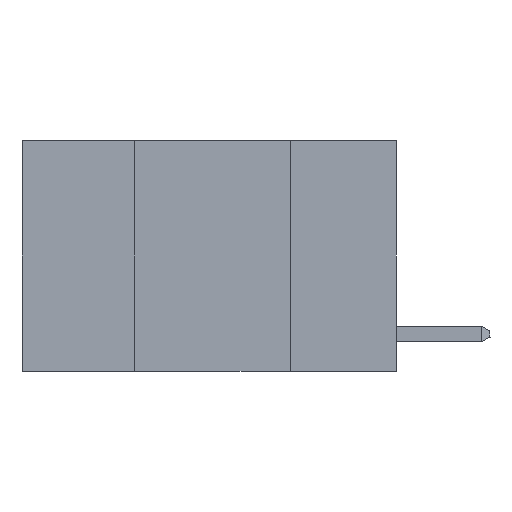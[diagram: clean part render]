
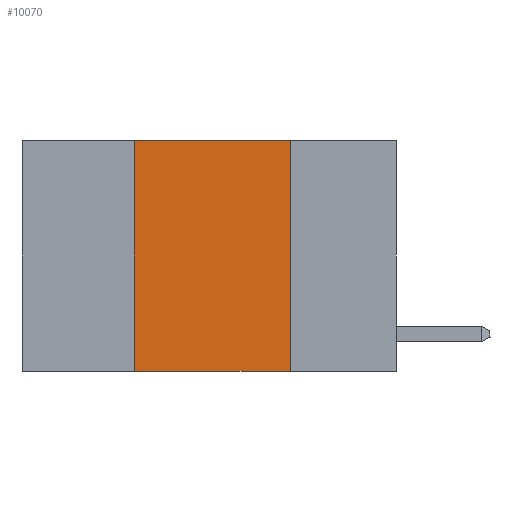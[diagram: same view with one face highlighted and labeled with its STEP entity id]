
A CAD part, left-side view. The second image highlights one B-rep face of the part: STEP entity #10070.
In plain terms, the highlighted planar face has unit normal (-1, 0, 0).
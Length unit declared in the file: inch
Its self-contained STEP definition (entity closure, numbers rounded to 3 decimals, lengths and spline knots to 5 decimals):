
#87 = EDGE_CURVE ( 'NONE', #2029, #4659, #8865, .T. ) ;
#155 = LINE ( 'NONE', #5042, #7788 ) ;
#282 = VERTEX_POINT ( 'NONE', #3450 ) ;
#465 = CARTESIAN_POINT ( 'NONE',  ( 0., 0.6, 0. ) ) ;
#720 = DIRECTION ( 'NONE',  ( 0., 0., -1. ) ) ;
#801 = VECTOR ( 'NONE', #3713, 39.37008 ) ;
#887 = ORIENTED_EDGE ( 'NONE', *, *, #6846, .T. ) ;
#1336 = LINE ( 'NONE', #10494, #801 ) ;
#1391 = DIRECTION ( 'NONE',  ( 0., -1., 0. ) ) ;
#1457 = DIRECTION ( 'NONE',  ( 0., 0., -1. ) ) ;
#1617 = VERTEX_POINT ( 'NONE', #4020 ) ;
#2029 = VERTEX_POINT ( 'NONE', #9677 ) ;
#2094 = LINE ( 'NONE', #465, #7392 ) ;
#2271 = FACE_OUTER_BOUND ( 'NONE', #10555, .T. ) ;
#2321 = CARTESIAN_POINT ( 'NONE',  ( 0., 0.6, 0. ) ) ;
#2398 = AXIS2_PLACEMENT_3D ( 'NONE', #2321, #5615, #1457 ) ;
#2466 = ORIENTED_EDGE ( 'NONE', *, *, #5228, .F. ) ;
#3450 = CARTESIAN_POINT ( 'NONE',  ( 0., 0.42, 0. ) ) ;
#3713 = DIRECTION ( 'NONE',  ( 0., -1., 0. ) ) ;
#4020 = CARTESIAN_POINT ( 'NONE',  ( 0., 0.42, -0.37 ) ) ;
#4296 = ORIENTED_EDGE ( 'NONE', *, *, #87, .F. ) ;
#4565 = ORIENTED_EDGE ( 'NONE', *, *, #6015, .F. ) ;
#4659 = VERTEX_POINT ( 'NONE', #7658 ) ;
#5005 = DIRECTION ( 'NONE',  ( 0., 0., 1. ) ) ;
#5042 = CARTESIAN_POINT ( 'NONE',  ( 0., 0.42, 0. ) ) ;
#5119 = VECTOR ( 'NONE', #720, 39.37008 ) ;
#5228 = EDGE_CURVE ( 'NONE', #282, #2029, #2094, .T. ) ;
#5615 = DIRECTION ( 'NONE',  ( 1., 0., 0. ) ) ;
#6015 = EDGE_CURVE ( 'NONE', #1617, #282, #155, .T. ) ;
#6846 = EDGE_CURVE ( 'NONE', #1617, #4659, #1336, .T. ) ;
#7392 = VECTOR ( 'NONE', #1391, 39.37008 ) ;
#7658 = CARTESIAN_POINT ( 'NONE',  ( 0., 0.17, -0.37 ) ) ;
#7788 = VECTOR ( 'NONE', #5005, 39.37008 ) ;
#8139 = PLANE ( 'NONE',  #2398 ) ;
#8865 = LINE ( 'NONE', #10407, #5119 ) ;
#9677 = CARTESIAN_POINT ( 'NONE',  ( 0., 0.17, 0. ) ) ;
#10070 = ADVANCED_FACE ( 'NONE', ( #2271 ), #8139, .F. ) ;
#10407 = CARTESIAN_POINT ( 'NONE',  ( 0., 0.17, 0. ) ) ;
#10494 = CARTESIAN_POINT ( 'NONE',  ( 0., 0.6, -0.37 ) ) ;
#10555 = EDGE_LOOP ( 'NONE', ( #4296, #2466, #4565, #887 ) ) ;
